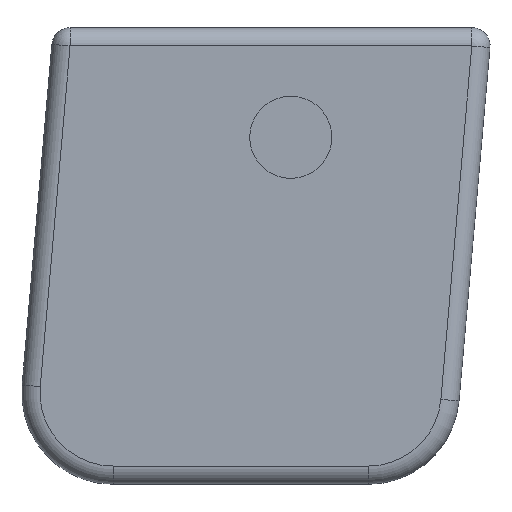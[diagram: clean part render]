
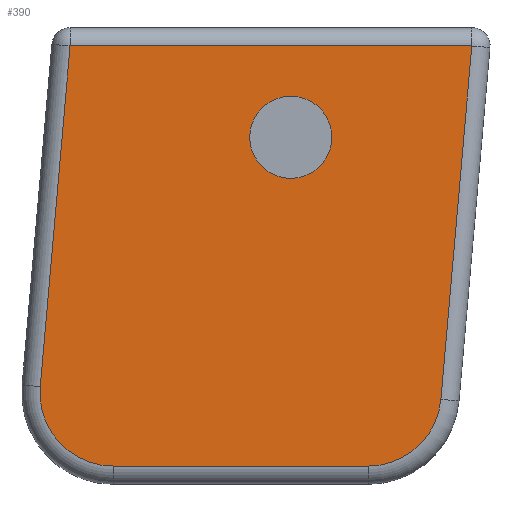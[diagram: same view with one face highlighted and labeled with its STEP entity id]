
A CAD part, front view. The second image highlights one B-rep face of the part: STEP entity #390.
In plain terms, the highlighted planar face has unit normal (0, -1, 0).
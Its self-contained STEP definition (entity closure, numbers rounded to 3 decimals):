
#15 = AXIS2_PLACEMENT_3D ( 'NONE', #31, #465, #97 ) ;
#16 = CARTESIAN_POINT ( 'NONE',  ( 9.493, 0., -14. ) ) ;
#31 = CARTESIAN_POINT ( 'NONE',  ( 4.911, 0., -10. ) ) ;
#36 = ORIENTED_EDGE ( 'NONE', *, *, #787, .F. ) ;
#59 = CARTESIAN_POINT ( 'NONE',  ( 9.727, 0., -0.851 ) ) ;
#60 = CIRCLE ( 'NONE', #569, 2.25 ) ;
#68 = VERTEX_POINT ( 'NONE', #237 ) ;
#75 = EDGE_LOOP ( 'NONE', ( #411, #680, #665, #642, #36, #181 ) ) ;
#94 = DIRECTION ( 'NONE',  ( 0., 1., 0. ) ) ;
#97 = DIRECTION ( 'NONE',  ( 0., 0., 1. ) ) ;
#109 = CARTESIAN_POINT ( 'NONE',  ( -9.051, 0., -10. ) ) ;
#124 = VERTEX_POINT ( 'NONE', #365 ) ;
#137 = EDGE_CURVE ( 'NONE', #364, #378, #456, .T. ) ;
#156 = VERTEX_POINT ( 'NONE', #756 ) ;
#181 = ORIENTED_EDGE ( 'NONE', *, *, #137, .T. ) ;
#182 = VECTOR ( 'NONE', #224, 1000. ) ;
#183 = DIRECTION ( 'NONE',  ( 0., 0., 1. ) ) ;
#191 = CARTESIAN_POINT ( 'NONE',  ( 0., 0., 9. ) ) ;
#193 = DIRECTION ( 'NONE',  ( 0., 1., 0. ) ) ;
#199 = CARTESIAN_POINT ( 'NONE',  ( -9.051, 0., -14. ) ) ;
#205 = DIRECTION ( 'NONE',  ( 0.087, 0., 0.996 ) ) ;
#206 = EDGE_CURVE ( 'NONE', #68, #624, #317, .T. ) ;
#222 = FACE_BOUND ( 'NONE', #345, .T. ) ;
#224 = DIRECTION ( 'NONE',  ( 1., 0., 0. ) ) ;
#237 = CARTESIAN_POINT ( 'NONE',  ( 0.68, 0., 6.25 ) ) ;
#282 = CARTESIAN_POINT ( 'NONE',  ( 0.68, 0., 1.75 ) ) ;
#286 = EDGE_CURVE ( 'NONE', #156, #484, #400, .T. ) ;
#303 = EDGE_CURVE ( 'NONE', #624, #68, #60, .T. ) ;
#309 = VERTEX_POINT ( 'NONE', #425 ) ;
#317 = CIRCLE ( 'NONE', #637, 2.25 ) ;
#320 = DIRECTION ( 'NONE',  ( 0., 0., 1. ) ) ;
#324 = LINE ( 'NONE', #59, #458 ) ;
#334 = LINE ( 'NONE', #695, #783 ) ;
#345 = EDGE_LOOP ( 'NONE', ( #435, #379 ) ) ;
#364 = VERTEX_POINT ( 'NONE', #199 ) ;
#365 = CARTESIAN_POINT ( 'NONE',  ( 8.896, 0., -10.349 ) ) ;
#378 = VERTEX_POINT ( 'NONE', #430 ) ;
#379 = ORIENTED_EDGE ( 'NONE', *, *, #303, .T. ) ;
#385 = VECTOR ( 'NONE', #779, 1000. ) ;
#390 = ADVANCED_FACE ( 'NONE', ( #222, #641 ), #555, .F. ) ;
#400 = LINE ( 'NONE', #191, #385 ) ;
#404 = EDGE_CURVE ( 'NONE', #124, #156, #324, .T. ) ;
#411 = ORIENTED_EDGE ( 'NONE', *, *, #711, .F. ) ;
#425 = CARTESIAN_POINT ( 'NONE',  ( -13.036, 0., -9.651 ) ) ;
#430 = CARTESIAN_POINT ( 'NONE',  ( 4.911, 0., -14. ) ) ;
#435 = ORIENTED_EDGE ( 'NONE', *, *, #206, .T. ) ;
#456 = LINE ( 'NONE', #16, #182 ) ;
#458 = VECTOR ( 'NONE', #205, 1000. ) ;
#464 = CARTESIAN_POINT ( 'NONE',  ( 0.68, 0., 4. ) ) ;
#465 = DIRECTION ( 'NONE',  ( 0., 1., 0. ) ) ;
#477 = AXIS2_PLACEMENT_3D ( 'NONE', #726, #676, #320 ) ;
#479 = AXIS2_PLACEMENT_3D ( 'NONE', #109, #535, #183 ) ;
#484 = VERTEX_POINT ( 'NONE', #623 ) ;
#512 = CIRCLE ( 'NONE', #479, 4. ) ;
#520 = DIRECTION ( 'NONE',  ( -0.087, 0., -0.996 ) ) ;
#523 = DIRECTION ( 'NONE',  ( 0., 0., 1. ) ) ;
#535 = DIRECTION ( 'NONE',  ( 0., 1., 0. ) ) ;
#545 = CARTESIAN_POINT ( 'NONE',  ( 0.68, 0., 4. ) ) ;
#555 = PLANE ( 'NONE',  #477 ) ;
#569 = AXIS2_PLACEMENT_3D ( 'NONE', #545, #193, #607 ) ;
#607 = DIRECTION ( 'NONE',  ( 0., 0., 1. ) ) ;
#623 = CARTESIAN_POINT ( 'NONE',  ( -11.404, 0., 9. ) ) ;
#624 = VERTEX_POINT ( 'NONE', #282 ) ;
#637 = AXIS2_PLACEMENT_3D ( 'NONE', #464, #94, #523 ) ;
#641 = FACE_OUTER_BOUND ( 'NONE', #75, .T. ) ;
#642 = ORIENTED_EDGE ( 'NONE', *, *, #675, .T. ) ;
#665 = ORIENTED_EDGE ( 'NONE', *, *, #286, .T. ) ;
#675 = EDGE_CURVE ( 'NONE', #484, #309, #334, .T. ) ;
#676 = DIRECTION ( 'NONE',  ( 0., 1., 0. ) ) ;
#680 = ORIENTED_EDGE ( 'NONE', *, *, #404, .T. ) ;
#695 = CARTESIAN_POINT ( 'NONE',  ( -13.511, 0., -15.087 ) ) ;
#711 = EDGE_CURVE ( 'NONE', #124, #378, #771, .T. ) ;
#726 = CARTESIAN_POINT ( 'NONE',  ( 0., 0., 0. ) ) ;
#756 = CARTESIAN_POINT ( 'NONE',  ( 10.588, 0., 9. ) ) ;
#771 = CIRCLE ( 'NONE', #15, 4. ) ;
#779 = DIRECTION ( 'NONE',  ( -1., 0., 0. ) ) ;
#783 = VECTOR ( 'NONE', #520, 1000. ) ;
#787 = EDGE_CURVE ( 'NONE', #364, #309, #512, .T. ) ;
